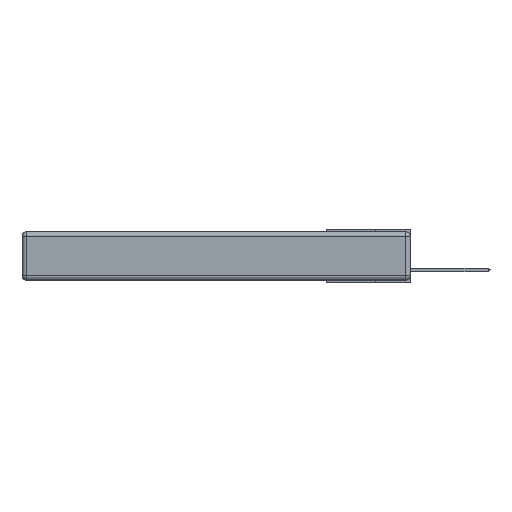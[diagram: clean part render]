
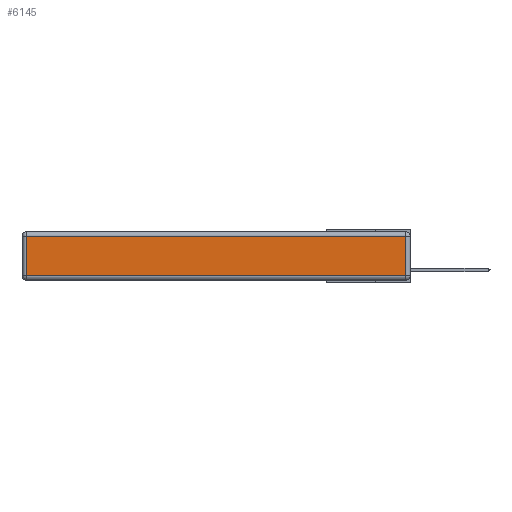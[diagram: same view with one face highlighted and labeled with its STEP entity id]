
A CAD part, left-side view. The second image highlights one B-rep face of the part: STEP entity #6145.
In plain terms, the highlighted planar face has unit normal (-1, 0, 0).
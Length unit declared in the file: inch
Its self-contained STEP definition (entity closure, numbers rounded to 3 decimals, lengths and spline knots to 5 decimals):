
#474 = CARTESIAN_POINT ( 'NONE',  ( 0., 2.72, -0.343 ) ) ;
#849 = EDGE_CURVE ( 'NONE', #6555, #6011, #22398, .T. ) ;
#1156 = DIRECTION ( 'NONE',  ( 0., 0., 1. ) ) ;
#2223 = EDGE_LOOP ( 'NONE', ( #7527, #3022, #21972, #11721 ) ) ;
#3022 = ORIENTED_EDGE ( 'NONE', *, *, #18261, .T. ) ;
#4865 = DIRECTION ( 'NONE',  ( 0., 0., -1. ) ) ;
#6011 = VERTEX_POINT ( 'NONE', #17342 ) ;
#6145 = ADVANCED_FACE ( 'NONE', ( #12858 ), #22203, .T. ) ;
#6262 = LINE ( 'NONE', #17530, #10038 ) ;
#6555 = VERTEX_POINT ( 'NONE', #23800 ) ;
#6997 = DIRECTION ( 'NONE',  ( -1., 0., 0. ) ) ;
#7527 = ORIENTED_EDGE ( 'NONE', *, *, #849, .T. ) ;
#7704 = LINE ( 'NONE', #474, #23030 ) ;
#10038 = VECTOR ( 'NONE', #1156, 39.37008 ) ;
#11721 = ORIENTED_EDGE ( 'NONE', *, *, #12647, .T. ) ;
#11914 = AXIS2_PLACEMENT_3D ( 'NONE', #17033, #6997, #18911 ) ;
#12581 = CARTESIAN_POINT ( 'NONE',  ( 0., 0.03, -0.03 ) ) ;
#12647 = EDGE_CURVE ( 'NONE', #16245, #6555, #7704, .T. ) ;
#12858 = FACE_OUTER_BOUND ( 'NONE', #2223, .T. ) ;
#14762 = VECTOR ( 'NONE', #23519, 39.37008 ) ;
#16099 = CARTESIAN_POINT ( 'NONE',  ( 0., 2.75, -0.03 ) ) ;
#16245 = VERTEX_POINT ( 'NONE', #17506 ) ;
#16718 = CARTESIAN_POINT ( 'NONE',  ( 0., 0., -0.313 ) ) ;
#17033 = CARTESIAN_POINT ( 'NONE',  ( 0., 0., -0.343 ) ) ;
#17342 = CARTESIAN_POINT ( 'NONE',  ( 0., 0.03, -0.313 ) ) ;
#17364 = LINE ( 'NONE', #16099, #14762 ) ;
#17506 = CARTESIAN_POINT ( 'NONE',  ( 0., 2.72, -0.03 ) ) ;
#17530 = CARTESIAN_POINT ( 'NONE',  ( 0., 0.03, -0.343 ) ) ;
#18193 = EDGE_CURVE ( 'NONE', #22741, #16245, #17364, .T. ) ;
#18261 = EDGE_CURVE ( 'NONE', #6011, #22741, #6262, .T. ) ;
#18911 = DIRECTION ( 'NONE',  ( 0., 0., 1. ) ) ;
#21972 = ORIENTED_EDGE ( 'NONE', *, *, #18193, .T. ) ;
#22203 = PLANE ( 'NONE',  #11914 ) ;
#22379 = DIRECTION ( 'NONE',  ( 0., -1., 0. ) ) ;
#22398 = LINE ( 'NONE', #16718, #23243 ) ;
#22741 = VERTEX_POINT ( 'NONE', #12581 ) ;
#23030 = VECTOR ( 'NONE', #4865, 39.37008 ) ;
#23243 = VECTOR ( 'NONE', #22379, 39.37008 ) ;
#23519 = DIRECTION ( 'NONE',  ( 0., 1., 0. ) ) ;
#23800 = CARTESIAN_POINT ( 'NONE',  ( 0., 2.72, -0.313 ) ) ;
